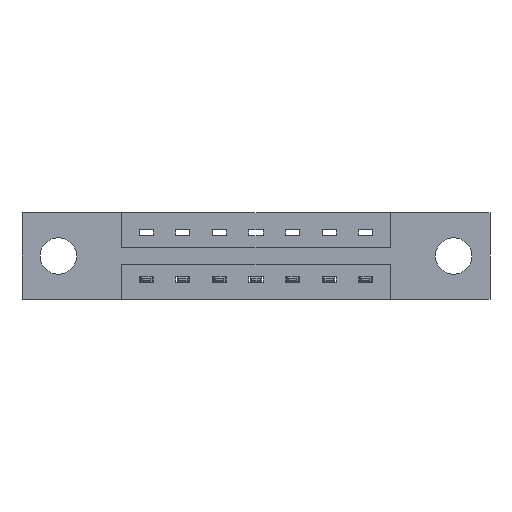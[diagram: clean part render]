
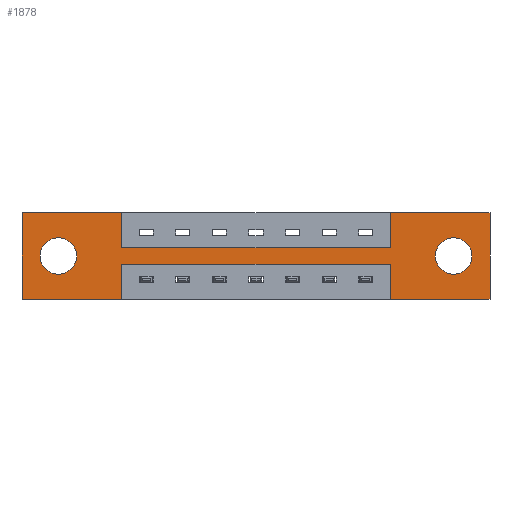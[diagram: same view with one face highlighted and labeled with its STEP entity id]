
A CAD part, front view. The second image highlights one B-rep face of the part: STEP entity #1878.
In plain terms, the highlighted planar face has unit normal (0, -1, 0).
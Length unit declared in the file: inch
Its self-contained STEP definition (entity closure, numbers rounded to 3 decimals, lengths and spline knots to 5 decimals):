
#26 = VERTEX_POINT ( 'NONE', #5701 ) ;
#65 = ORIENTED_EDGE ( 'NONE', *, *, #2620, .F. ) ;
#80 = ORIENTED_EDGE ( 'NONE', *, *, #6548, .F. ) ;
#225 = VERTEX_POINT ( 'NONE', #5803 ) ;
#235 = CIRCLE ( 'NONE', #6271, 0.078 ) ;
#324 = CARTESIAN_POINT ( 'NONE',  ( 1.843, 0., -0.263 ) ) ;
#429 = VERTEX_POINT ( 'NONE', #8804 ) ;
#439 = CARTESIAN_POINT ( 'NONE',  ( 1.573, 0., -0.37 ) ) ;
#599 = CIRCLE ( 'NONE', #8153, 0.078 ) ;
#620 = DIRECTION ( 'NONE',  ( 0., 0., 1. ) ) ;
#708 = ORIENTED_EDGE ( 'NONE', *, *, #2397, .T. ) ;
#810 = CARTESIAN_POINT ( 'NONE',  ( 0., 0., 0. ) ) ;
#877 = CARTESIAN_POINT ( 'NONE',  ( 1.998, 0., 0. ) ) ;
#907 = EDGE_CURVE ( 'NONE', #1149, #8682, #2255, .T. ) ;
#961 = CARTESIAN_POINT ( 'NONE',  ( 0., 0., 0. ) ) ;
#969 = DIRECTION ( 'NONE',  ( 1., 0., 0. ) ) ;
#973 = LINE ( 'NONE', #961, #5224 ) ;
#980 = VERTEX_POINT ( 'NONE', #324 ) ;
#1060 = DIRECTION ( 'NONE',  ( 0., 1., 0. ) ) ;
#1149 = VERTEX_POINT ( 'NONE', #1255 ) ;
#1151 = LINE ( 'NONE', #439, #8711 ) ;
#1185 = LINE ( 'NONE', #8878, #4943 ) ;
#1255 = CARTESIAN_POINT ( 'NONE',  ( 0.155, 0., -0.263 ) ) ;
#1319 = VECTOR ( 'NONE', #7049, 39.37008 ) ;
#1413 = CARTESIAN_POINT ( 'NONE',  ( 1.998, 0., -0.37 ) ) ;
#1543 = ORIENTED_EDGE ( 'NONE', *, *, #8694, .F. ) ;
#1574 = DIRECTION ( 'NONE',  ( 0., 0., -1. ) ) ;
#1586 = EDGE_CURVE ( 'NONE', #4900, #6004, #1185, .T. ) ;
#1689 = VERTEX_POINT ( 'NONE', #8505 ) ;
#1878 = ADVANCED_FACE ( 'NONE', ( #8419, #2775, #3012 ), #4575, .T. ) ;
#1973 = ORIENTED_EDGE ( 'NONE', *, *, #6967, .F. ) ;
#2047 = CARTESIAN_POINT ( 'NONE',  ( 0., 0., -0.37 ) ) ;
#2156 = CARTESIAN_POINT ( 'NONE',  ( 0.425, 0., -0.15 ) ) ;
#2249 = CARTESIAN_POINT ( 'NONE',  ( 0.425, 0., -0.37 ) ) ;
#2255 = CIRCLE ( 'NONE', #5569, 0.078 ) ;
#2263 = CIRCLE ( 'NONE', #4385, 0.078 ) ;
#2338 = VERTEX_POINT ( 'NONE', #7914 ) ;
#2397 = EDGE_CURVE ( 'NONE', #8682, #1149, #235, .T. ) ;
#2430 = EDGE_CURVE ( 'NONE', #4328, #2338, #7993, .T. ) ;
#2448 = AXIS2_PLACEMENT_3D ( 'NONE', #2800, #3454, #3475 ) ;
#2590 = DIRECTION ( 'NONE',  ( 1., 0., 0. ) ) ;
#2620 = EDGE_CURVE ( 'NONE', #8051, #5393, #8297, .T. ) ;
#2640 = CARTESIAN_POINT ( 'NONE',  ( 0., 0., 0. ) ) ;
#2740 = VECTOR ( 'NONE', #969, 39.37008 ) ;
#2775 = FACE_BOUND ( 'NONE', #9004, .T. ) ;
#2800 = CARTESIAN_POINT ( 'NONE',  ( 0., 0., -0.37 ) ) ;
#2891 = DIRECTION ( 'NONE',  ( -1., 0., 0. ) ) ;
#2917 = ORIENTED_EDGE ( 'NONE', *, *, #1586, .F. ) ;
#2958 = CARTESIAN_POINT ( 'NONE',  ( 0., 0., -0.37 ) ) ;
#3012 = FACE_OUTER_BOUND ( 'NONE', #7233, .T. ) ;
#3015 = CARTESIAN_POINT ( 'NONE',  ( 1.573, 0., 0. ) ) ;
#3145 = ORIENTED_EDGE ( 'NONE', *, *, #6737, .F. ) ;
#3146 = CARTESIAN_POINT ( 'NONE',  ( 0., 0., 0. ) ) ;
#3153 = EDGE_CURVE ( 'NONE', #5393, #429, #7294, .T. ) ;
#3187 = ORIENTED_EDGE ( 'NONE', *, *, #8531, .F. ) ;
#3235 = ORIENTED_EDGE ( 'NONE', *, *, #3818, .F. ) ;
#3303 = LINE ( 'NONE', #8165, #6918 ) ;
#3454 = DIRECTION ( 'NONE',  ( 0., -1., 0. ) ) ;
#3475 = DIRECTION ( 'NONE',  ( 0., 0., -1. ) ) ;
#3655 = DIRECTION ( 'NONE',  ( -1., 0., 0. ) ) ;
#3818 = EDGE_CURVE ( 'NONE', #2338, #8810, #5702, .T. ) ;
#4025 = ORIENTED_EDGE ( 'NONE', *, *, #907, .T. ) ;
#4081 = VECTOR ( 'NONE', #6398, 39.37008 ) ;
#4113 = CARTESIAN_POINT ( 'NONE',  ( 0.425, 0., -0.22 ) ) ;
#4328 = VERTEX_POINT ( 'NONE', #5144 ) ;
#4385 = AXIS2_PLACEMENT_3D ( 'NONE', #7003, #6949, #6938 ) ;
#4520 = ORIENTED_EDGE ( 'NONE', *, *, #5771, .T. ) ;
#4544 = ORIENTED_EDGE ( 'NONE', *, *, #3153, .F. ) ;
#4575 = PLANE ( 'NONE',  #2448 ) ;
#4601 = VERTEX_POINT ( 'NONE', #8830 ) ;
#4761 = CARTESIAN_POINT ( 'NONE',  ( 0.425, 0., 0. ) ) ;
#4771 = LINE ( 'NONE', #2640, #2740 ) ;
#4853 = VECTOR ( 'NONE', #2590, 39.37008 ) ;
#4900 = VERTEX_POINT ( 'NONE', #877 ) ;
#4902 = VECTOR ( 'NONE', #2891, 39.37008 ) ;
#4943 = VECTOR ( 'NONE', #9436, 39.37008 ) ;
#5109 = LINE ( 'NONE', #3146, #4853 ) ;
#5144 = CARTESIAN_POINT ( 'NONE',  ( 0.425, 0., -0.15 ) ) ;
#5224 = VECTOR ( 'NONE', #5827, 39.37008 ) ;
#5229 = DIRECTION ( 'NONE',  ( 0., 0., 1. ) ) ;
#5279 = VECTOR ( 'NONE', #3655, 39.37008 ) ;
#5294 = ORIENTED_EDGE ( 'NONE', *, *, #7821, .T. ) ;
#5338 = VERTEX_POINT ( 'NONE', #810 ) ;
#5341 = EDGE_CURVE ( 'NONE', #1689, #4601, #1151, .T. ) ;
#5393 = VERTEX_POINT ( 'NONE', #2249 ) ;
#5567 = ORIENTED_EDGE ( 'NONE', *, *, #5341, .F. ) ;
#5569 = AXIS2_PLACEMENT_3D ( 'NONE', #9496, #9442, #5680 ) ;
#5633 = LINE ( 'NONE', #4761, #7229 ) ;
#5680 = DIRECTION ( 'NONE',  ( 0., 0., 1. ) ) ;
#5701 = CARTESIAN_POINT ( 'NONE',  ( 1.843, 0., -0.107 ) ) ;
#5702 = LINE ( 'NONE', #6446, #1319 ) ;
#5771 = EDGE_CURVE ( 'NONE', #26, #980, #599, .T. ) ;
#5803 = CARTESIAN_POINT ( 'NONE',  ( 0.425, 0., 0. ) ) ;
#5827 = DIRECTION ( 'NONE',  ( 0., 0., 1. ) ) ;
#5852 = DIRECTION ( 'NONE',  ( 0., 0., -1. ) ) ;
#5887 = DIRECTION ( 'NONE',  ( 0., 1., 0. ) ) ;
#6004 = VERTEX_POINT ( 'NONE', #1413 ) ;
#6049 = CARTESIAN_POINT ( 'NONE',  ( 1.843, 0., -0.185 ) ) ;
#6271 = AXIS2_PLACEMENT_3D ( 'NONE', #8740, #1060, #5229 ) ;
#6294 = ORIENTED_EDGE ( 'NONE', *, *, #7107, .F. ) ;
#6398 = DIRECTION ( 'NONE',  ( 1., 0., 0. ) ) ;
#6446 = CARTESIAN_POINT ( 'NONE',  ( 1.573, 0., 0. ) ) ;
#6520 = CARTESIAN_POINT ( 'NONE',  ( 0.155, 0., -0.107 ) ) ;
#6548 = EDGE_CURVE ( 'NONE', #4601, #8051, #3303, .T. ) ;
#6555 = VECTOR ( 'NONE', #7334, 39.37008 ) ;
#6737 = EDGE_CURVE ( 'NONE', #429, #5338, #973, .T. ) ;
#6901 = ORIENTED_EDGE ( 'NONE', *, *, #2430, .F. ) ;
#6918 = VECTOR ( 'NONE', #8449, 39.37008 ) ;
#6938 = DIRECTION ( 'NONE',  ( 0., 0., -1. ) ) ;
#6949 = DIRECTION ( 'NONE',  ( 0., 1., 0. ) ) ;
#6967 = EDGE_CURVE ( 'NONE', #8810, #4900, #5109, .T. ) ;
#7003 = CARTESIAN_POINT ( 'NONE',  ( 1.843, 0., -0.185 ) ) ;
#7018 = CARTESIAN_POINT ( 'NONE',  ( 0.425, 0., -0.37 ) ) ;
#7049 = DIRECTION ( 'NONE',  ( 0., 0., 1. ) ) ;
#7107 = EDGE_CURVE ( 'NONE', #225, #4328, #5633, .T. ) ;
#7229 = VECTOR ( 'NONE', #1574, 39.37008 ) ;
#7233 = EDGE_LOOP ( 'NONE', ( #65, #80, #5567, #1543, #2917, #1973, #3235, #6901, #6294, #3187, #3145, #4544 ) ) ;
#7294 = LINE ( 'NONE', #2958, #5279 ) ;
#7334 = DIRECTION ( 'NONE',  ( 0., 0., -1. ) ) ;
#7629 = EDGE_LOOP ( 'NONE', ( #4520, #5294 ) ) ;
#7821 = EDGE_CURVE ( 'NONE', #980, #26, #2263, .T. ) ;
#7914 = CARTESIAN_POINT ( 'NONE',  ( 1.573, 0., -0.15 ) ) ;
#7993 = LINE ( 'NONE', #2156, #4081 ) ;
#8051 = VERTEX_POINT ( 'NONE', #4113 ) ;
#8153 = AXIS2_PLACEMENT_3D ( 'NONE', #6049, #5887, #5852 ) ;
#8165 = CARTESIAN_POINT ( 'NONE',  ( 0.425, 0., -0.22 ) ) ;
#8297 = LINE ( 'NONE', #7018, #6555 ) ;
#8419 = FACE_BOUND ( 'NONE', #7629, .T. ) ;
#8449 = DIRECTION ( 'NONE',  ( -1., 0., 0. ) ) ;
#8503 = LINE ( 'NONE', #2047, #4902 ) ;
#8505 = CARTESIAN_POINT ( 'NONE',  ( 1.573, 0., -0.37 ) ) ;
#8531 = EDGE_CURVE ( 'NONE', #5338, #225, #4771, .T. ) ;
#8682 = VERTEX_POINT ( 'NONE', #6520 ) ;
#8694 = EDGE_CURVE ( 'NONE', #6004, #1689, #8503, .T. ) ;
#8711 = VECTOR ( 'NONE', #620, 39.37008 ) ;
#8740 = CARTESIAN_POINT ( 'NONE',  ( 0.155, 0., -0.185 ) ) ;
#8804 = CARTESIAN_POINT ( 'NONE',  ( 0., 0., -0.37 ) ) ;
#8810 = VERTEX_POINT ( 'NONE', #3015 ) ;
#8830 = CARTESIAN_POINT ( 'NONE',  ( 1.573, 0., -0.22 ) ) ;
#8878 = CARTESIAN_POINT ( 'NONE',  ( 1.998, 0., 0. ) ) ;
#9004 = EDGE_LOOP ( 'NONE', ( #708, #4025 ) ) ;
#9436 = DIRECTION ( 'NONE',  ( 0., 0., -1. ) ) ;
#9442 = DIRECTION ( 'NONE',  ( 0., 1., 0. ) ) ;
#9496 = CARTESIAN_POINT ( 'NONE',  ( 0.155, 0., -0.185 ) ) ;
